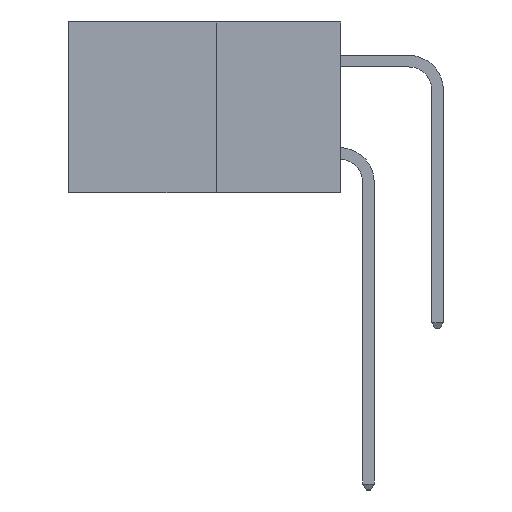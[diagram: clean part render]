
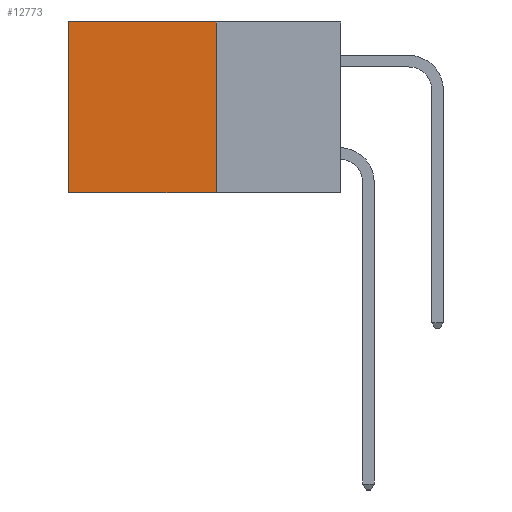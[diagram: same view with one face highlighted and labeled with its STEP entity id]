
A CAD part, left-side view. The second image highlights one B-rep face of the part: STEP entity #12773.
In plain terms, the highlighted planar face has unit normal (-1, 0, 0).
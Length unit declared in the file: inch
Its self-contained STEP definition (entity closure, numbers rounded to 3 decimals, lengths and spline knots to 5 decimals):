
#31 = AXIS2_PLACEMENT_3D ( 'NONE', #10663, #5619, #12687 ) ;
#400 = ORIENTED_EDGE ( 'NONE', *, *, #6570, .T. ) ;
#597 = CARTESIAN_POINT ( 'NONE',  ( 0.277, 0.59, 0. ) ) ;
#888 = CARTESIAN_POINT ( 'NONE',  ( 0.277, 0.59, -0.37 ) ) ;
#1460 = EDGE_CURVE ( 'NONE', #7876, #3129, #2021, .T. ) ;
#1667 = VECTOR ( 'NONE', #5788, 39.37008 ) ;
#2021 = LINE ( 'NONE', #7086, #7092 ) ;
#3129 = VERTEX_POINT ( 'NONE', #597 ) ;
#4092 = VECTOR ( 'NONE', #9102, 39.37008 ) ;
#4463 = VECTOR ( 'NONE', #7932, 39.37008 ) ;
#5238 = ORIENTED_EDGE ( 'NONE', *, *, #1460, .T. ) ;
#5619 = DIRECTION ( 'NONE',  ( 1., 0., 0. ) ) ;
#5788 = DIRECTION ( 'NONE',  ( 0., 1., 0. ) ) ;
#5842 = CARTESIAN_POINT ( 'NONE',  ( 0.277, 0.27, -0.37 ) ) ;
#6169 = ORIENTED_EDGE ( 'NONE', *, *, #11620, .F. ) ;
#6570 = EDGE_CURVE ( 'NONE', #3129, #13162, #6979, .T. ) ;
#6976 = LINE ( 'NONE', #5842, #4463 ) ;
#6979 = LINE ( 'NONE', #12044, #4092 ) ;
#7086 = CARTESIAN_POINT ( 'NONE',  ( 0.277, 0.27, 0. ) ) ;
#7092 = VECTOR ( 'NONE', #11482, 39.37008 ) ;
#7414 = VERTEX_POINT ( 'NONE', #10352 ) ;
#7801 = CARTESIAN_POINT ( 'NONE',  ( 0.277, 0.27, -0.37 ) ) ;
#7805 = EDGE_LOOP ( 'NONE', ( #400, #9379, #6169, #5238 ) ) ;
#7876 = VERTEX_POINT ( 'NONE', #11275 ) ;
#7932 = DIRECTION ( 'NONE',  ( 0., 0., -1. ) ) ;
#9102 = DIRECTION ( 'NONE',  ( 0., 0., -1. ) ) ;
#9379 = ORIENTED_EDGE ( 'NONE', *, *, #13327, .F. ) ;
#9736 = PLANE ( 'NONE',  #31 ) ;
#10140 = LINE ( 'NONE', #7801, #1667 ) ;
#10318 = FACE_OUTER_BOUND ( 'NONE', #7805, .T. ) ;
#10352 = CARTESIAN_POINT ( 'NONE',  ( 0.277, 0.27, -0.37 ) ) ;
#10663 = CARTESIAN_POINT ( 'NONE',  ( 0.277, 0.27, -0.37 ) ) ;
#11275 = CARTESIAN_POINT ( 'NONE',  ( 0.277, 0.27, 0. ) ) ;
#11482 = DIRECTION ( 'NONE',  ( 0., 1., 0. ) ) ;
#11620 = EDGE_CURVE ( 'NONE', #7876, #7414, #6976, .T. ) ;
#12044 = CARTESIAN_POINT ( 'NONE',  ( 0.277, 0.59, -0.37 ) ) ;
#12687 = DIRECTION ( 'NONE',  ( 0., 0., -1. ) ) ;
#12773 = ADVANCED_FACE ( 'NONE', ( #10318 ), #9736, .F. ) ;
#13162 = VERTEX_POINT ( 'NONE', #888 ) ;
#13327 = EDGE_CURVE ( 'NONE', #7414, #13162, #10140, .T. ) ;
